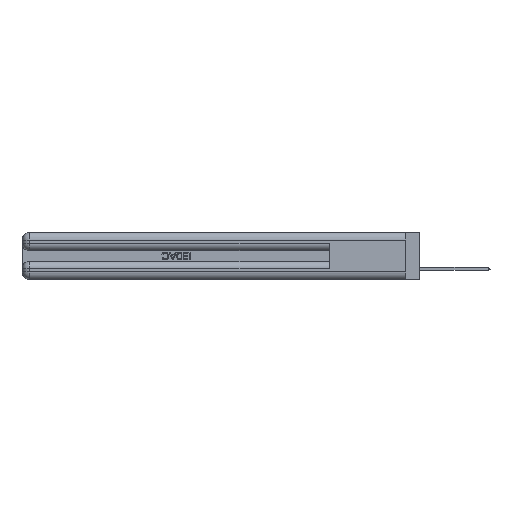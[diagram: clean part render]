
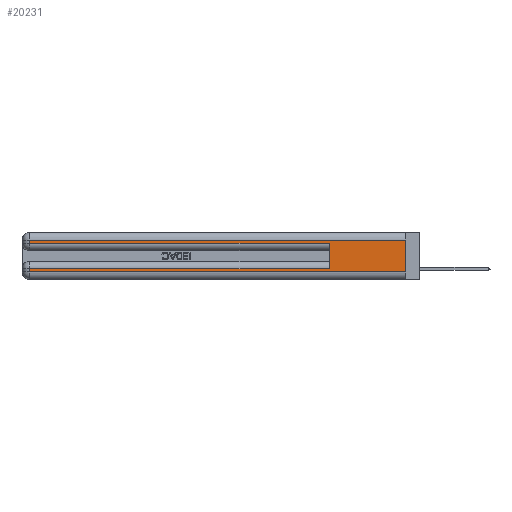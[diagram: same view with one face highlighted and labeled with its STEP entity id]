
A CAD part, left-side view. The second image highlights one B-rep face of the part: STEP entity #20231.
In plain terms, the highlighted planar face has unit normal (-1, 0, 0).
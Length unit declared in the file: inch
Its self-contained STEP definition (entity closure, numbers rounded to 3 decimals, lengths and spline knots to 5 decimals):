
#155 = EDGE_CURVE ( 'NONE', #50789, #18745, #2116, .T. ) ;
#659 = ORIENTED_EDGE ( 'NONE', *, *, #43104, .T. ) ;
#1079 = CARTESIAN_POINT ( 'NONE',  ( 0., 2.94, 0.37 ) ) ;
#1626 = VECTOR ( 'NONE', #49289, 39.37008 ) ;
#2116 = LINE ( 'NONE', #28709, #43429 ) ;
#2252 = CARTESIAN_POINT ( 'NONE',  ( 0., 2.94, 0.06 ) ) ;
#2452 = LINE ( 'NONE', #25167, #16888 ) ;
#2816 = EDGE_CURVE ( 'NONE', #50957, #11865, #19959, .T. ) ;
#3024 = DIRECTION ( 'NONE',  ( 0., 0., -1. ) ) ;
#3314 = CARTESIAN_POINT ( 'NONE',  ( 0., 0., 0.31 ) ) ;
#3709 = LINE ( 'NONE', #11413, #7455 ) ;
#4196 = DIRECTION ( 'NONE',  ( 0., 0., 1. ) ) ;
#6405 = VERTEX_POINT ( 'NONE', #30834 ) ;
#7455 = VECTOR ( 'NONE', #39426, 39.37008 ) ;
#9239 = VECTOR ( 'NONE', #9288, 39.37008 ) ;
#9288 = DIRECTION ( 'NONE',  ( 0., -1., 0. ) ) ;
#10105 = CARTESIAN_POINT ( 'NONE',  ( 0., 0., 0.085 ) ) ;
#11413 = CARTESIAN_POINT ( 'NONE',  ( 0., 0., 0.285 ) ) ;
#11865 = VERTEX_POINT ( 'NONE', #31809 ) ;
#15875 = VECTOR ( 'NONE', #42833, 39.37008 ) ;
#16888 = VECTOR ( 'NONE', #17106, 39.37008 ) ;
#17106 = DIRECTION ( 'NONE',  ( 0., 1., 0. ) ) ;
#18711 = ORIENTED_EDGE ( 'NONE', *, *, #38611, .F. ) ;
#18745 = VERTEX_POINT ( 'NONE', #33473 ) ;
#18993 = LINE ( 'NONE', #50874, #15875 ) ;
#19045 = FACE_OUTER_BOUND ( 'NONE', #40771, .T. ) ;
#19312 = VECTOR ( 'NONE', #51697, 39.37008 ) ;
#19959 = LINE ( 'NONE', #29296, #9239 ) ;
#20231 = ADVANCED_FACE ( 'NONE', ( #19045 ), #22308, .F. ) ;
#21706 = LINE ( 'NONE', #10105, #1626 ) ;
#22308 = PLANE ( 'NONE',  #29167 ) ;
#25150 = ORIENTED_EDGE ( 'NONE', *, *, #45702, .T. ) ;
#25167 = CARTESIAN_POINT ( 'NONE',  ( 0., 0., 0.31 ) ) ;
#25601 = CARTESIAN_POINT ( 'NONE',  ( 0., 2.94, 0.085 ) ) ;
#28709 = CARTESIAN_POINT ( 'NONE',  ( 0., 0.6, 0.145 ) ) ;
#29167 = AXIS2_PLACEMENT_3D ( 'NONE', #43405, #50911, #3024 ) ;
#29296 = CARTESIAN_POINT ( 'NONE',  ( 0., 0., 0.06 ) ) ;
#30341 = ORIENTED_EDGE ( 'NONE', *, *, #44660, .T. ) ;
#30834 = CARTESIAN_POINT ( 'NONE',  ( 0., 2.94, 0.31 ) ) ;
#31809 = CARTESIAN_POINT ( 'NONE',  ( 0., 0., 0.06 ) ) ;
#33473 = CARTESIAN_POINT ( 'NONE',  ( 0., 0.6, 0.285 ) ) ;
#33702 = ORIENTED_EDGE ( 'NONE', *, *, #155, .F. ) ;
#35629 = VERTEX_POINT ( 'NONE', #47555 ) ;
#37560 = CARTESIAN_POINT ( 'NONE',  ( 0., 0.6, 0.085 ) ) ;
#38611 = EDGE_CURVE ( 'NONE', #49132, #11865, #18993, .T. ) ;
#39048 = VECTOR ( 'NONE', #41109, 39.37008 ) ;
#39426 = DIRECTION ( 'NONE',  ( 0., -1., 0. ) ) ;
#40331 = EDGE_CURVE ( 'NONE', #35629, #18745, #3709, .T. ) ;
#40446 = LINE ( 'NONE', #47731, #19312 ) ;
#40771 = EDGE_LOOP ( 'NONE', ( #18711, #659, #45491, #47750, #33702, #25150, #30341, #46160 ) ) ;
#41109 = DIRECTION ( 'NONE',  ( 0., 0., -1. ) ) ;
#41503 = LINE ( 'NONE', #1079, #39048 ) ;
#42833 = DIRECTION ( 'NONE',  ( 0., 0., -1. ) ) ;
#43104 = EDGE_CURVE ( 'NONE', #49132, #6405, #2452, .T. ) ;
#43405 = CARTESIAN_POINT ( 'NONE',  ( 0., 0., 0.37 ) ) ;
#43429 = VECTOR ( 'NONE', #4196, 39.37008 ) ;
#44660 = EDGE_CURVE ( 'NONE', #47090, #50957, #40446, .T. ) ;
#45491 = ORIENTED_EDGE ( 'NONE', *, *, #47027, .T. ) ;
#45702 = EDGE_CURVE ( 'NONE', #50789, #47090, #21706, .T. ) ;
#46160 = ORIENTED_EDGE ( 'NONE', *, *, #2816, .T. ) ;
#47027 = EDGE_CURVE ( 'NONE', #6405, #35629, #41503, .T. ) ;
#47090 = VERTEX_POINT ( 'NONE', #25601 ) ;
#47555 = CARTESIAN_POINT ( 'NONE',  ( 0., 2.94, 0.285 ) ) ;
#47731 = CARTESIAN_POINT ( 'NONE',  ( 0., 2.94, 0.37 ) ) ;
#47750 = ORIENTED_EDGE ( 'NONE', *, *, #40331, .T. ) ;
#49132 = VERTEX_POINT ( 'NONE', #3314 ) ;
#49289 = DIRECTION ( 'NONE',  ( 0., 1., 0. ) ) ;
#50789 = VERTEX_POINT ( 'NONE', #37560 ) ;
#50874 = CARTESIAN_POINT ( 'NONE',  ( 0., 0., 0.37 ) ) ;
#50911 = DIRECTION ( 'NONE',  ( 1., 0., 0. ) ) ;
#50957 = VERTEX_POINT ( 'NONE', #2252 ) ;
#51697 = DIRECTION ( 'NONE',  ( 0., 0., -1. ) ) ;
